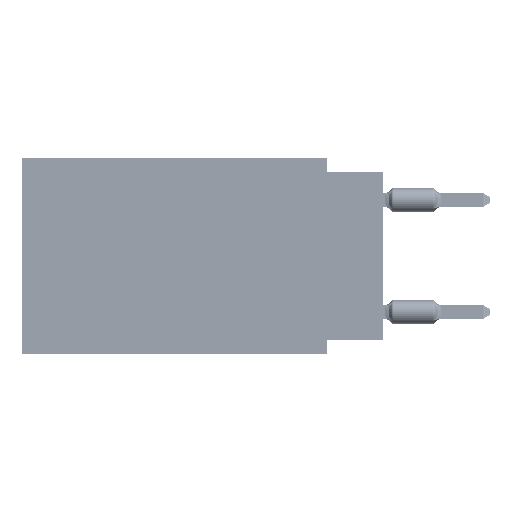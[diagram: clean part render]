
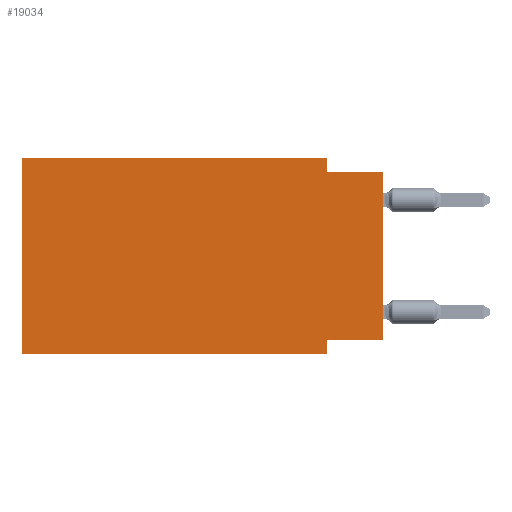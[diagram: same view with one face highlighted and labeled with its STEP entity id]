
A CAD part, left-side view. The second image highlights one B-rep face of the part: STEP entity #19034.
In plain terms, the highlighted planar face has unit normal (-1, 0, 0).
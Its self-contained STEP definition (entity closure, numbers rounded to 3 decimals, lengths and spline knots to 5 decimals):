
#206 = VERTEX_POINT ( 'NONE', #30516 ) ;
#1266 = ORIENTED_EDGE ( 'NONE', *, *, #53879, .F. ) ;
#1281 = CARTESIAN_POINT ( 'NONE',  ( 0., 0.645, 0. ) ) ;
#1951 = DIRECTION ( 'NONE',  ( 0., 1., 0. ) ) ;
#2854 = CARTESIAN_POINT ( 'NONE',  ( 0., 0.645, 0. ) ) ;
#3218 = DIRECTION ( 'NONE',  ( 0., -1., 0. ) ) ;
#3245 = VECTOR ( 'NONE', #62994, 39.37008 ) ;
#5167 = ORIENTED_EDGE ( 'NONE', *, *, #65450, .F. ) ;
#6078 = VERTEX_POINT ( 'NONE', #1281 ) ;
#7632 = DIRECTION ( 'NONE',  ( 1., 0., 0. ) ) ;
#11470 = CARTESIAN_POINT ( 'NONE',  ( 0., 0.1, -0.35 ) ) ;
#15044 = LINE ( 'NONE', #2854, #59104 ) ;
#16474 = CARTESIAN_POINT ( 'NONE',  ( 0., 0., -0.025 ) ) ;
#19034 = ADVANCED_FACE ( 'NONE', ( #82930 ), #58928, .F. ) ;
#19286 = LINE ( 'NONE', #44925, #58385 ) ;
#19802 = DIRECTION ( 'NONE',  ( 0., -1., 0. ) ) ;
#23791 = LINE ( 'NONE', #60819, #64176 ) ;
#25493 = VERTEX_POINT ( 'NONE', #16474 ) ;
#27922 = EDGE_CURVE ( 'NONE', #6078, #72177, #45841, .T. ) ;
#28060 = DIRECTION ( 'NONE',  ( 0., 0., 1. ) ) ;
#29436 = CARTESIAN_POINT ( 'NONE',  ( 0., 0.645, -0.35 ) ) ;
#30516 = CARTESIAN_POINT ( 'NONE',  ( 0., 0.1, -0.325 ) ) ;
#33224 = LINE ( 'NONE', #79034, #44054 ) ;
#33502 = LINE ( 'NONE', #58334, #68470 ) ;
#37121 = DIRECTION ( 'NONE',  ( 0., 0., -1. ) ) ;
#37782 = CARTESIAN_POINT ( 'NONE',  ( 0., 0.1, 0. ) ) ;
#39586 = CARTESIAN_POINT ( 'NONE',  ( 0., 0.645, 0. ) ) ;
#41275 = CARTESIAN_POINT ( 'NONE',  ( 0., 0., -0.325 ) ) ;
#44054 = VECTOR ( 'NONE', #58876, 39.37008 ) ;
#44925 = CARTESIAN_POINT ( 'NONE',  ( 0., 0., 0. ) ) ;
#45841 = LINE ( 'NONE', #77408, #66939 ) ;
#46015 = ORIENTED_EDGE ( 'NONE', *, *, #48471, .F. ) ;
#48471 = EDGE_CURVE ( 'NONE', #72177, #78384, #76886, .T. ) ;
#49914 = VECTOR ( 'NONE', #37121, 39.37008 ) ;
#49965 = AXIS2_PLACEMENT_3D ( 'NONE', #39586, #7632, #76638 ) ;
#50148 = LINE ( 'NONE', #11470, #49914 ) ;
#50394 = DIRECTION ( 'NONE',  ( 0., 0., 1. ) ) ;
#52409 = CARTESIAN_POINT ( 'NONE',  ( 0., 0.1, 0. ) ) ;
#53879 = EDGE_CURVE ( 'NONE', #78384, #25493, #23791, .T. ) ;
#54538 = EDGE_CURVE ( 'NONE', #81111, #77101, #33224, .T. ) ;
#56661 = EDGE_CURVE ( 'NONE', #69707, #206, #33502, .T. ) ;
#58334 = CARTESIAN_POINT ( 'NONE',  ( 0., 0., -0.325 ) ) ;
#58385 = VECTOR ( 'NONE', #50394, 39.37008 ) ;
#58876 = DIRECTION ( 'NONE',  ( 0., -1., 0. ) ) ;
#58928 = PLANE ( 'NONE',  #49965 ) ;
#59104 = VECTOR ( 'NONE', #28060, 39.37008 ) ;
#60819 = CARTESIAN_POINT ( 'NONE',  ( 0., 0., -0.025 ) ) ;
#62246 = ORIENTED_EDGE ( 'NONE', *, *, #56661, .F. ) ;
#62833 = CARTESIAN_POINT ( 'NONE',  ( 0., 0.1, -0.35 ) ) ;
#62994 = DIRECTION ( 'NONE',  ( 0., 0., -1. ) ) ;
#64176 = VECTOR ( 'NONE', #3218, 39.37008 ) ;
#65450 = EDGE_CURVE ( 'NONE', #206, #77101, #50148, .T. ) ;
#66939 = VECTOR ( 'NONE', #19802, 39.37008 ) ;
#68470 = VECTOR ( 'NONE', #1951, 39.37008 ) ;
#69707 = VERTEX_POINT ( 'NONE', #41275 ) ;
#70406 = EDGE_CURVE ( 'NONE', #69707, #25493, #19286, .T. ) ;
#72177 = VERTEX_POINT ( 'NONE', #52409 ) ;
#72388 = EDGE_LOOP ( 'NONE', ( #72432, #1266, #46015, #78894, #80361, #75402, #5167, #62246 ) ) ;
#72432 = ORIENTED_EDGE ( 'NONE', *, *, #70406, .T. ) ;
#75402 = ORIENTED_EDGE ( 'NONE', *, *, #54538, .T. ) ;
#76638 = DIRECTION ( 'NONE',  ( 0., 0., -1. ) ) ;
#76886 = LINE ( 'NONE', #37782, #3245 ) ;
#77101 = VERTEX_POINT ( 'NONE', #62833 ) ;
#77408 = CARTESIAN_POINT ( 'NONE',  ( 0., 0.645, 0. ) ) ;
#78223 = EDGE_CURVE ( 'NONE', #81111, #6078, #15044, .T. ) ;
#78384 = VERTEX_POINT ( 'NONE', #80636 ) ;
#78894 = ORIENTED_EDGE ( 'NONE', *, *, #27922, .F. ) ;
#79034 = CARTESIAN_POINT ( 'NONE',  ( 0., 0.645, -0.35 ) ) ;
#80361 = ORIENTED_EDGE ( 'NONE', *, *, #78223, .F. ) ;
#80636 = CARTESIAN_POINT ( 'NONE',  ( 0., 0.1, -0.025 ) ) ;
#81111 = VERTEX_POINT ( 'NONE', #29436 ) ;
#82930 = FACE_OUTER_BOUND ( 'NONE', #72388, .T. ) ;
